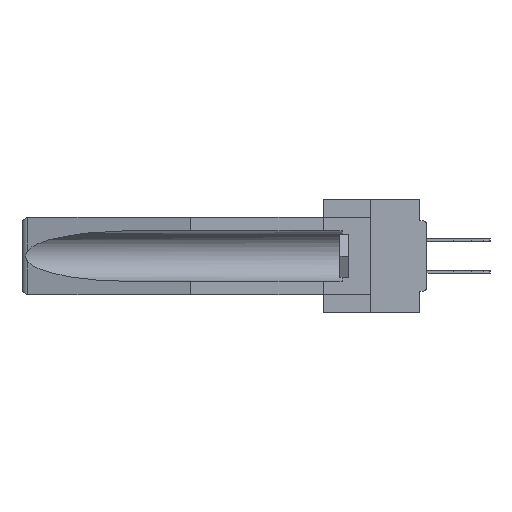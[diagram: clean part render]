
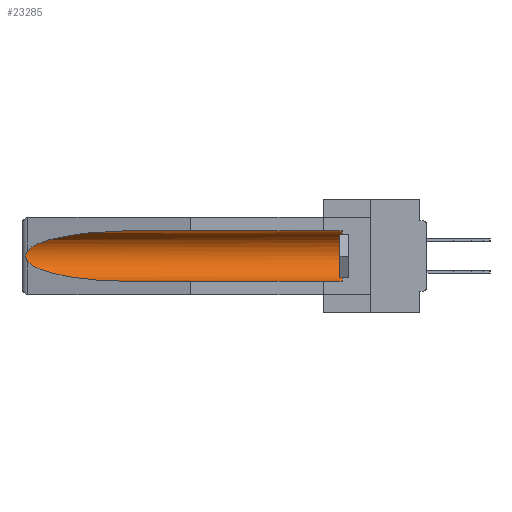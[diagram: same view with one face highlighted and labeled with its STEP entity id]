
A CAD part, left-side view. The second image highlights one B-rep face of the part: STEP entity #23285.
In plain terms, the highlighted cylindrical face has radius 2.857 mm (diameter 5.715 mm), a partial arc.
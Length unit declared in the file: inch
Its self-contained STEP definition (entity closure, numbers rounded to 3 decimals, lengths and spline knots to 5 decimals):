
#102 = EDGE_CURVE ( 'NONE', #31562, #36422, #31999, .T. ) ;
#1682 = CARTESIAN_POINT ( 'NONE',  ( 0.26655, 1.53094, -0.18657 ) ) ;
#3261 = EDGE_LOOP ( 'NONE', ( #20095, #14403, #20425, #9819, #30767, #41839 ) ) ;
#4285 = CARTESIAN_POINT ( 'NONE',  ( 0.26537, 1.52718, -0.19328 ) ) ;
#4647 = DIRECTION ( 'NONE',  ( 0., -1., 0. ) ) ;
#5001 = EDGE_CURVE ( 'NONE', #17020, #26796, #9899, .T. ) ;
#5033 = FACE_OUTER_BOUND ( 'NONE', #3261, .T. ) ;
#5488 = CARTESIAN_POINT ( 'NONE',  ( 0.2675, 1.53308, -0.16763 ) ) ;
#6597 = CARTESIAN_POINT ( 'NONE',  ( 0.26537, 1.52718, -0.19328 ) ) ;
#7867 = EDGE_CURVE ( 'NONE', #14610, #14890, #23271, .T. ) ;
#8637 = CARTESIAN_POINT ( 'NONE',  ( 0.26537, 1.52718, -0.19328 ) ) ;
#9819 = ORIENTED_EDGE ( 'NONE', *, *, #12320, .F. ) ;
#9899 =( BOUNDED_CURVE ( )  B_SPLINE_CURVE ( 3, ( #40938, #34418, #31013, #24407 ),
 .UNSPECIFIED., .F., .F. ) 
 B_SPLINE_CURVE_WITH_KNOTS ( ( 4, 4 ),
 ( 4.71239, 6.08839 ),
 .UNSPECIFIED. ) 
 CURVE ( )  GEOMETRIC_REPRESENTATION_ITEM ( )  RATIONAL_B_SPLINE_CURVE ( ( 1., 0.848, 0.848, 1. ) ) 
 REPRESENTATION_ITEM ( '' )  );
#12254 = DIRECTION ( 'NONE',  ( 0., 1., 0. ) ) ;
#12320 = EDGE_CURVE ( 'NONE', #31562, #14890, #35600, .T. ) ;
#12358 = DIRECTION ( 'NONE',  ( 0., 1., 0. ) ) ;
#14403 = ORIENTED_EDGE ( 'NONE', *, *, #36790, .T. ) ;
#14610 = VERTEX_POINT ( 'NONE', #6597 ) ;
#14777 = CARTESIAN_POINT ( 'NONE',  ( 0.26537, 1.52718, -0.14972 ) ) ;
#14890 = VERTEX_POINT ( 'NONE', #25879 ) ;
#15318 = CARTESIAN_POINT ( 'NONE',  ( 0.155, 1.07973, -0.059 ) ) ;
#15858 = B_SPLINE_CURVE_WITH_KNOTS ( 'NONE', 3,
 ( #22181, #22334, #29547, #42749, #5488, #39030, #29254, #1682, #25778, #8637 ),
 .UNSPECIFIED., .F., .F.,
 ( 4, 2, 2, 2, 4 ),
 ( 0., 0.00029, 0.00058, 0.00087, 0.00117 ),
 .UNSPECIFIED. ) ;
#16020 = CARTESIAN_POINT ( 'NONE',  ( 0.155, 0.126, -0.059 ) ) ;
#16781 = EDGE_CURVE ( 'NONE', #36422, #17020, #17764, .T. ) ;
#17020 = VERTEX_POINT ( 'NONE', #15318 ) ;
#17329 = CYLINDRICAL_SURFACE ( 'NONE', #24325, 0.1125 ) ;
#17764 = LINE ( 'NONE', #36367, #22551 ) ;
#18006 = CARTESIAN_POINT ( 'NONE',  ( 0.25451, 1.48313, -0.24835 ) ) ;
#18827 = AXIS2_PLACEMENT_3D ( 'NONE', #41798, #4647, #35423 ) ;
#20095 = ORIENTED_EDGE ( 'NONE', *, *, #5001, .T. ) ;
#20425 = ORIENTED_EDGE ( 'NONE', *, *, #7867, .T. ) ;
#22181 = CARTESIAN_POINT ( 'NONE',  ( 0.26537, 1.52718, -0.14972 ) ) ;
#22334 = CARTESIAN_POINT ( 'NONE',  ( 0.26597, 1.52961, -0.15275 ) ) ;
#22551 = VECTOR ( 'NONE', #32644, 39.37008 ) ;
#22665 = CARTESIAN_POINT ( 'NONE',  ( 0.155, -0.30754, -0.284 ) ) ;
#23271 =( BOUNDED_CURVE ( )  B_SPLINE_CURVE ( 3, ( #4285, #18006, #35194, #34896 ),
 .UNSPECIFIED., .F., .F. ) 
 B_SPLINE_CURVE_WITH_KNOTS ( ( 4, 4 ),
 ( 0.1948, 1.5708 ),
 .UNSPECIFIED. ) 
 CURVE ( )  GEOMETRIC_REPRESENTATION_ITEM ( )  RATIONAL_B_SPLINE_CURVE ( ( 1., 0.848, 0.848, 1. ) ) 
 REPRESENTATION_ITEM ( '' )  );
#23285 = ADVANCED_FACE ( 'NONE', ( #5033 ), #17329, .F. ) ;
#24325 = AXIS2_PLACEMENT_3D ( 'NONE', #42971, #12254, #36010 ) ;
#24407 = CARTESIAN_POINT ( 'NONE',  ( 0.26537, 1.52718, -0.14972 ) ) ;
#25778 = CARTESIAN_POINT ( 'NONE',  ( 0.26597, 1.5296, -0.19026 ) ) ;
#25879 = CARTESIAN_POINT ( 'NONE',  ( 0.155, 1.07973, -0.284 ) ) ;
#26796 = VERTEX_POINT ( 'NONE', #14777 ) ;
#29254 = CARTESIAN_POINT ( 'NONE',  ( 0.2673, 1.53269, -0.17917 ) ) ;
#29547 = CARTESIAN_POINT ( 'NONE',  ( 0.26654, 1.53092, -0.15636 ) ) ;
#30767 = ORIENTED_EDGE ( 'NONE', *, *, #102, .T. ) ;
#31013 = CARTESIAN_POINT ( 'NONE',  ( 0.25451, 1.48313, -0.09465 ) ) ;
#31562 = VERTEX_POINT ( 'NONE', #34686 ) ;
#31999 = CIRCLE ( 'NONE', #18827, 0.1125 ) ;
#32644 = DIRECTION ( 'NONE',  ( 0., 1., 0. ) ) ;
#34418 = CARTESIAN_POINT ( 'NONE',  ( 0.21114, 1.30732, -0.059 ) ) ;
#34686 = CARTESIAN_POINT ( 'NONE',  ( 0.155, 0.126, -0.284 ) ) ;
#34896 = CARTESIAN_POINT ( 'NONE',  ( 0.155, 1.07973, -0.284 ) ) ;
#35194 = CARTESIAN_POINT ( 'NONE',  ( 0.21114, 1.30732, -0.284 ) ) ;
#35423 = DIRECTION ( 'NONE',  ( 0., 0., 1. ) ) ;
#35600 = LINE ( 'NONE', #22665, #41968 ) ;
#36010 = DIRECTION ( 'NONE',  ( 0., 0., 1. ) ) ;
#36367 = CARTESIAN_POINT ( 'NONE',  ( 0.155, -0.30754, -0.059 ) ) ;
#36422 = VERTEX_POINT ( 'NONE', #16020 ) ;
#36790 = EDGE_CURVE ( 'NONE', #26796, #14610, #15858, .T. ) ;
#39030 = CARTESIAN_POINT ( 'NONE',  ( 0.2675, 1.53308, -0.17534 ) ) ;
#40938 = CARTESIAN_POINT ( 'NONE',  ( 0.155, 1.07973, -0.059 ) ) ;
#41798 = CARTESIAN_POINT ( 'NONE',  ( 0.155, 0.126, -0.1715 ) ) ;
#41839 = ORIENTED_EDGE ( 'NONE', *, *, #16781, .T. ) ;
#41968 = VECTOR ( 'NONE', #12358, 39.37008 ) ;
#42749 = CARTESIAN_POINT ( 'NONE',  ( 0.2673, 1.5327, -0.16383 ) ) ;
#42971 = CARTESIAN_POINT ( 'NONE',  ( 0.155, -0.30754, -0.1715 ) ) ;
